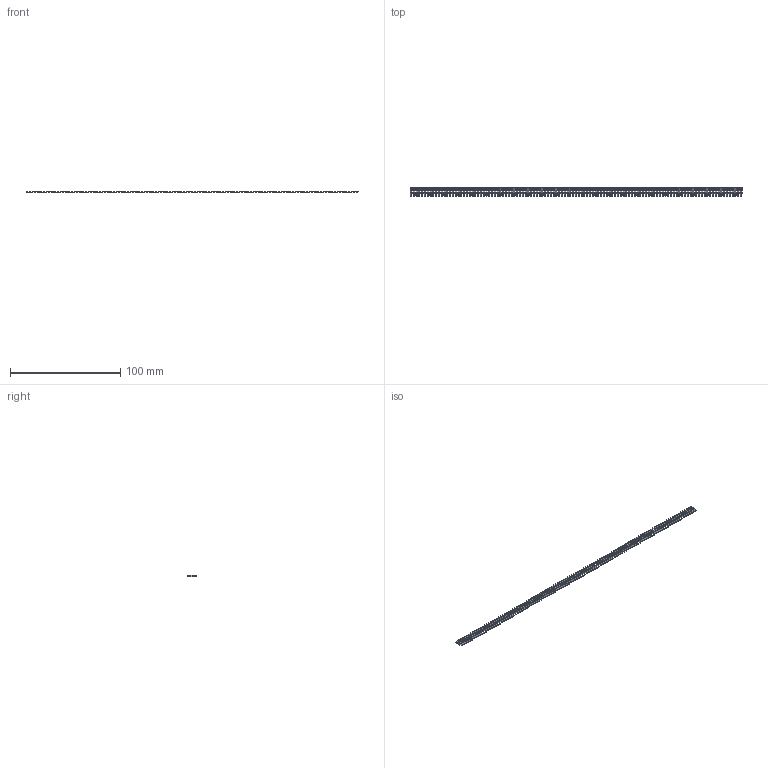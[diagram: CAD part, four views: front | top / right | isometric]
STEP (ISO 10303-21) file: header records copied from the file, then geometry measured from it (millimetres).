
FILE_DESCRIPTION (( 'STEP AP203' ), '1' );
FILE_NAME ('106-119-253-100.STEP', '2020-04-16T23:43:32', ( '' ), ( '' ), 'SwSTEP 2.0', 'SolidWorks 2016', '' );
FILE_SCHEMA (( 'CONFIG_CONTROL_DESIGN' ));
Length unit declared in the file: inch
Products named in the file (2): 100-290-001_100-290-253; 106-119-253-100
Assembly tree (119 placements, depth 2):
  106-119-253-100
    100-290-001_100-290-253  x119
Bounding box: 301.52 x 7.62 x 1.8 mm (x, y, z)
Volume: 656.6 mm3; surface area: 4094.4 mm2
Topology: 119 solids, 119 shells, 2380 faces, 6426 edges, 4284 vertices
Faces by surface type: plane 2261, cylinder 119
Entity records: 4596 total; most frequent: DIRECTION 340, CALENDAR_DATE 248, DATE_AND_TIME 248, COORDINATED_UNIVERSAL_TIME_OFFSET 248, LOCAL_TIME 248, CARTESIAN_POINT 232, AXIS2_PLACEMENT_3D 144, PERSON_AND_ORGANIZATION 135
